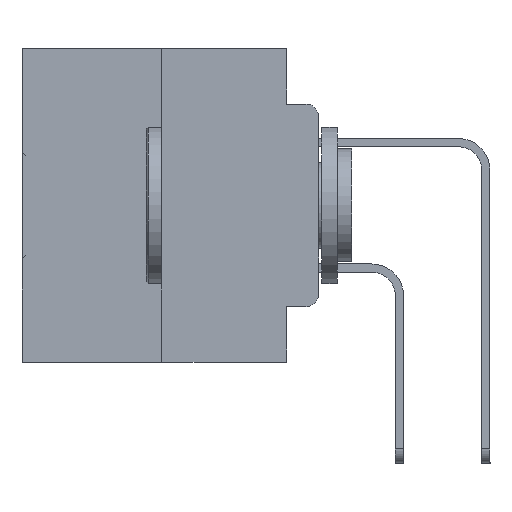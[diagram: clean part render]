
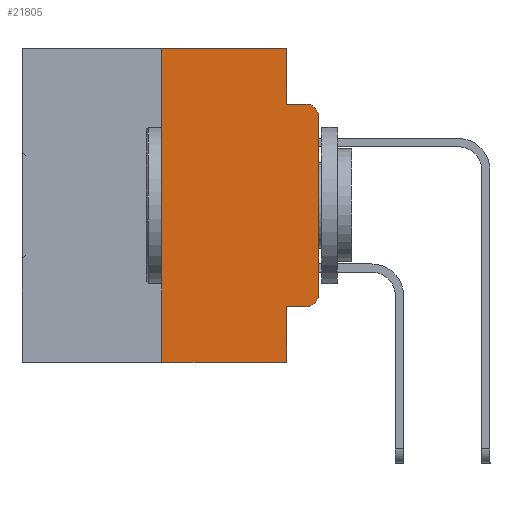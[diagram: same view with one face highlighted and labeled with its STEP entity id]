
A CAD part, left-side view. The second image highlights one B-rep face of the part: STEP entity #21805.
In plain terms, the highlighted planar face has unit normal (-1, 0, 0).
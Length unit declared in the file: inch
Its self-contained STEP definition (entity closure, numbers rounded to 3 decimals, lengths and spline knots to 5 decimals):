
#420 = VERTEX_POINT ( 'NONE', #11479 ) ;
#606 = DIRECTION ( 'NONE',  ( 0., 0., 1. ) ) ;
#644 = CARTESIAN_POINT ( 'NONE',  ( 0., 0., 0. ) ) ;
#1073 = CARTESIAN_POINT ( 'NONE',  ( 0., 0.051, -0.4115 ) ) ;
#1577 = EDGE_CURVE ( 'NONE', #31001, #8367, #6773, .T. ) ;
#1765 = LINE ( 'NONE', #6497, #32633 ) ;
#1802 = VERTEX_POINT ( 'NONE', #22206 ) ;
#1879 = VECTOR ( 'NONE', #606, 39.37008 ) ;
#2274 = CARTESIAN_POINT ( 'NONE',  ( 0., 0.051, -0.0885 ) ) ;
#2335 = CARTESIAN_POINT ( 'NONE',  ( 0., 0.051, -0.4115 ) ) ;
#3052 = EDGE_CURVE ( 'NONE', #420, #8418, #9034, .T. ) ;
#3864 = VECTOR ( 'NONE', #32900, 39.37008 ) ;
#4111 = LINE ( 'NONE', #12106, #18182 ) ;
#4906 = CARTESIAN_POINT ( 'NONE',  ( 0., 0.25, -0.5 ) ) ;
#4947 = LINE ( 'NONE', #24055, #9564 ) ;
#5857 = EDGE_CURVE ( 'NONE', #27302, #17446, #17942, .T. ) ;
#5952 = DIRECTION ( 'NONE',  ( -1., 0., 0. ) ) ;
#6185 = CARTESIAN_POINT ( 'NONE',  ( 0., 0.25, 0. ) ) ;
#6411 = CARTESIAN_POINT ( 'NONE',  ( 0., 0., -0.1085 ) ) ;
#6497 = CARTESIAN_POINT ( 'NONE',  ( 0., 0.051, -0.0885 ) ) ;
#6773 = LINE ( 'NONE', #33232, #19967 ) ;
#6775 = VERTEX_POINT ( 'NONE', #2274 ) ;
#6896 = ORIENTED_EDGE ( 'NONE', *, *, #10902, .F. ) ;
#6987 = CARTESIAN_POINT ( 'NONE',  ( 0., 0.051, 0. ) ) ;
#8367 = VERTEX_POINT ( 'NONE', #6185 ) ;
#8418 = VERTEX_POINT ( 'NONE', #6411 ) ;
#8565 = ORIENTED_EDGE ( 'NONE', *, *, #11547, .T. ) ;
#8677 = VECTOR ( 'NONE', #30337, 39.37008 ) ;
#8902 = CARTESIAN_POINT ( 'NONE',  ( 0., 0.02, -0.1085 ) ) ;
#9034 = LINE ( 'NONE', #644, #1879 ) ;
#9178 = DIRECTION ( 'NONE',  ( 0., 0., 1. ) ) ;
#9219 = DIRECTION ( 'NONE',  ( 0., -1., 0. ) ) ;
#9564 = VECTOR ( 'NONE', #16232, 39.37008 ) ;
#9823 = ORIENTED_EDGE ( 'NONE', *, *, #28388, .T. ) ;
#10120 = EDGE_CURVE ( 'NONE', #27302, #15518, #33689, .T. ) ;
#10423 = DIRECTION ( 'NONE',  ( 0., -1., 0. ) ) ;
#10902 = EDGE_CURVE ( 'NONE', #8367, #1802, #4947, .T. ) ;
#11052 = ORIENTED_EDGE ( 'NONE', *, *, #32281, .T. ) ;
#11442 = ORIENTED_EDGE ( 'NONE', *, *, #27325, .F. ) ;
#11479 = CARTESIAN_POINT ( 'NONE',  ( 0., 0., -0.3915 ) ) ;
#11542 = DIRECTION ( 'NONE',  ( 0., 0., -1. ) ) ;
#11547 = EDGE_CURVE ( 'NONE', #31001, #17446, #4111, .T. ) ;
#11825 = CIRCLE ( 'NONE', #15938, 0.02 ) ;
#12106 = CARTESIAN_POINT ( 'NONE',  ( 0., 0.473, -0.5 ) ) ;
#12637 = DIRECTION ( 'NONE',  ( 0., 0., -1. ) ) ;
#12664 = CARTESIAN_POINT ( 'NONE',  ( 0., 0.02, -0.4115 ) ) ;
#12959 = FACE_OUTER_BOUND ( 'NONE', #27825, .T. ) ;
#13643 = VERTEX_POINT ( 'NONE', #25869 ) ;
#13895 = ORIENTED_EDGE ( 'NONE', *, *, #1577, .F. ) ;
#15518 = VERTEX_POINT ( 'NONE', #12664 ) ;
#15689 = LINE ( 'NONE', #6987, #8677 ) ;
#15938 = AXIS2_PLACEMENT_3D ( 'NONE', #21723, #5952, #24304 ) ;
#16232 = DIRECTION ( 'NONE',  ( 0., -1., 0. ) ) ;
#16392 = ORIENTED_EDGE ( 'NONE', *, *, #10120, .T. ) ;
#17292 = AXIS2_PLACEMENT_3D ( 'NONE', #30558, #28175, #12637 ) ;
#17446 = VERTEX_POINT ( 'NONE', #31735 ) ;
#17942 = LINE ( 'NONE', #33328, #3864 ) ;
#18182 = VECTOR ( 'NONE', #30149, 39.37008 ) ;
#19464 = CIRCLE ( 'NONE', #24369, 0.02 ) ;
#19967 = VECTOR ( 'NONE', #9178, 39.37008 ) ;
#21723 = CARTESIAN_POINT ( 'NONE',  ( 0., 0.02, -0.3915 ) ) ;
#21805 = ADVANCED_FACE ( 'NONE', ( #12959 ), #23054, .F. ) ;
#22081 = ORIENTED_EDGE ( 'NONE', *, *, #3052, .T. ) ;
#22206 = CARTESIAN_POINT ( 'NONE',  ( 0., 0.051, 0. ) ) ;
#23054 = PLANE ( 'NONE',  #17292 ) ;
#24055 = CARTESIAN_POINT ( 'NONE',  ( 0., 0.473, 0. ) ) ;
#24304 = DIRECTION ( 'NONE',  ( 0., 0., -1. ) ) ;
#24369 = AXIS2_PLACEMENT_3D ( 'NONE', #8902, #27105, #11542 ) ;
#25869 = CARTESIAN_POINT ( 'NONE',  ( 0., 0.02, -0.0885 ) ) ;
#27105 = DIRECTION ( 'NONE',  ( -1., 0., 0. ) ) ;
#27302 = VERTEX_POINT ( 'NONE', #1073 ) ;
#27325 = EDGE_CURVE ( 'NONE', #6775, #13643, #1765, .T. ) ;
#27825 = EDGE_LOOP ( 'NONE', ( #22081, #9823, #11442, #31957, #6896, #13895, #8565, #29256, #16392, #11052 ) ) ;
#28175 = DIRECTION ( 'NONE',  ( 1., 0., 0. ) ) ;
#28388 = EDGE_CURVE ( 'NONE', #8418, #13643, #19464, .T. ) ;
#29256 = ORIENTED_EDGE ( 'NONE', *, *, #5857, .F. ) ;
#29617 = EDGE_CURVE ( 'NONE', #1802, #6775, #15689, .T. ) ;
#30149 = DIRECTION ( 'NONE',  ( 0., -1., 0. ) ) ;
#30337 = DIRECTION ( 'NONE',  ( 0., 0., -1. ) ) ;
#30558 = CARTESIAN_POINT ( 'NONE',  ( 0., 0.473, 0. ) ) ;
#31001 = VERTEX_POINT ( 'NONE', #4906 ) ;
#31735 = CARTESIAN_POINT ( 'NONE',  ( 0., 0.051, -0.5 ) ) ;
#31957 = ORIENTED_EDGE ( 'NONE', *, *, #29617, .F. ) ;
#32281 = EDGE_CURVE ( 'NONE', #15518, #420, #11825, .T. ) ;
#32633 = VECTOR ( 'NONE', #9219, 39.37008 ) ;
#32900 = DIRECTION ( 'NONE',  ( 0., 0., -1. ) ) ;
#32924 = VECTOR ( 'NONE', #10423, 39.37008 ) ;
#33232 = CARTESIAN_POINT ( 'NONE',  ( 0., 0.25, 0. ) ) ;
#33328 = CARTESIAN_POINT ( 'NONE',  ( 0., 0.051, 0. ) ) ;
#33689 = LINE ( 'NONE', #2335, #32924 ) ;
